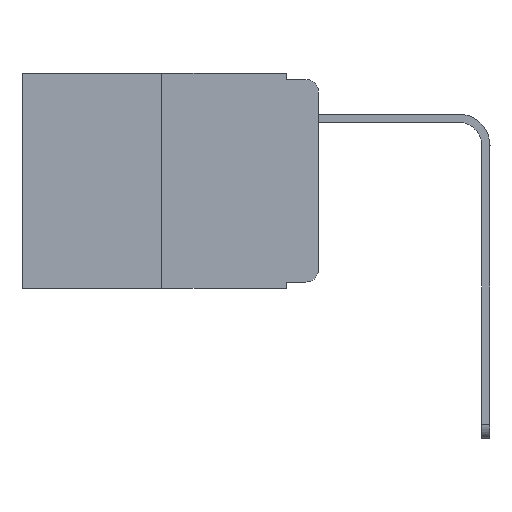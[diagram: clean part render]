
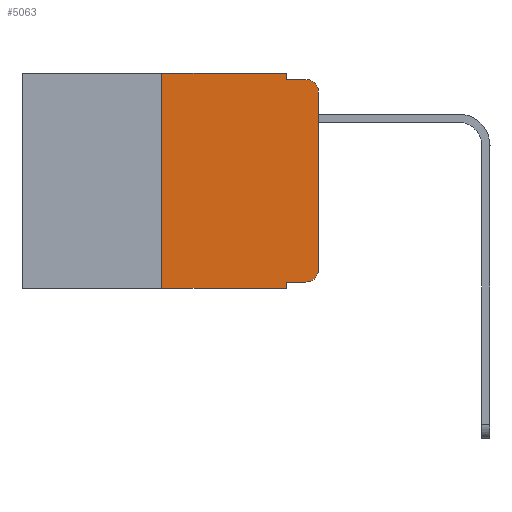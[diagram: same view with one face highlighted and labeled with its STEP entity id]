
A CAD part, left-side view. The second image highlights one B-rep face of the part: STEP entity #5063.
In plain terms, the highlighted planar face has unit normal (-1, 0, 0).
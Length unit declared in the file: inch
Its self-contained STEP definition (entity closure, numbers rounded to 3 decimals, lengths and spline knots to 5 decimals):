
#220 = CARTESIAN_POINT ( 'NONE',  ( 0., 0.25, 0. ) ) ;
#316 = DIRECTION ( 'NONE',  ( 0., 0., -1. ) ) ;
#384 = ORIENTED_EDGE ( 'NONE', *, *, #5271, .F. ) ;
#535 = VERTEX_POINT ( 'NONE', #10327 ) ;
#571 = EDGE_CURVE ( 'NONE', #6502, #5930, #3643, .T. ) ;
#575 = ORIENTED_EDGE ( 'NONE', *, *, #2331, .F. ) ;
#621 = DIRECTION ( 'NONE',  ( 0., 0., 1. ) ) ;
#719 = DIRECTION ( 'NONE',  ( -1., 0., 0. ) ) ;
#898 = CARTESIAN_POINT ( 'NONE',  ( 0., 0., -0.03 ) ) ;
#991 = EDGE_CURVE ( 'NONE', #1486, #1157, #9545, .T. ) ;
#1157 = VERTEX_POINT ( 'NONE', #9462 ) ;
#1486 = VERTEX_POINT ( 'NONE', #9009 ) ;
#1503 = CARTESIAN_POINT ( 'NONE',  ( 0., 0.473, 0. ) ) ;
#1522 = ORIENTED_EDGE ( 'NONE', *, *, #10848, .T. ) ;
#1525 = AXIS2_PLACEMENT_3D ( 'NONE', #6087, #719, #6989 ) ;
#1906 = VECTOR ( 'NONE', #10087, 39.37008 ) ;
#1943 = CIRCLE ( 'NONE', #1525, 0.02 ) ;
#1952 = ORIENTED_EDGE ( 'NONE', *, *, #8018, .F. ) ;
#2265 = EDGE_LOOP ( 'NONE', ( #9313, #9713, #575, #384, #1952, #3880, #11541, #6491, #1522, #4829 ) ) ;
#2331 = EDGE_CURVE ( 'NONE', #7788, #9104, #4872, .T. ) ;
#2636 = VECTOR ( 'NONE', #10453, 39.37008 ) ;
#2656 = VECTOR ( 'NONE', #4838, 39.37008 ) ;
#2702 = PLANE ( 'NONE',  #6130 ) ;
#3017 = VERTEX_POINT ( 'NONE', #6590 ) ;
#3643 = LINE ( 'NONE', #5897, #4207 ) ;
#3785 = CARTESIAN_POINT ( 'NONE',  ( 0., 0., 0. ) ) ;
#3832 = EDGE_CURVE ( 'NONE', #1157, #10319, #10558, .T. ) ;
#3880 = ORIENTED_EDGE ( 'NONE', *, *, #571, .F. ) ;
#3940 = CARTESIAN_POINT ( 'NONE',  ( 0., 0.051, -0.01 ) ) ;
#4207 = VECTOR ( 'NONE', #621, 39.37008 ) ;
#4244 = VECTOR ( 'NONE', #10772, 39.37008 ) ;
#4511 = CARTESIAN_POINT ( 'NONE',  ( 0., 0.02, -0.01 ) ) ;
#4617 = FACE_OUTER_BOUND ( 'NONE', #2265, .T. ) ;
#4671 = VECTOR ( 'NONE', #11520, 39.37008 ) ;
#4796 = CARTESIAN_POINT ( 'NONE',  ( 0., 0.02, -0.313 ) ) ;
#4829 = ORIENTED_EDGE ( 'NONE', *, *, #991, .T. ) ;
#4838 = DIRECTION ( 'NONE',  ( 0., 0., -1. ) ) ;
#4872 = LINE ( 'NONE', #3940, #9363 ) ;
#5039 = AXIS2_PLACEMENT_3D ( 'NONE', #4796, #9378, #316 ) ;
#5063 = ADVANCED_FACE ( 'NONE', ( #4617 ), #2702, .F. ) ;
#5271 = EDGE_CURVE ( 'NONE', #6372, #7788, #7131, .T. ) ;
#5481 = DIRECTION ( 'NONE',  ( 1., 0., 0. ) ) ;
#5635 = CARTESIAN_POINT ( 'NONE',  ( 0., 0.051, -0.01 ) ) ;
#5897 = CARTESIAN_POINT ( 'NONE',  ( 0., 0.25, 0. ) ) ;
#5930 = VERTEX_POINT ( 'NONE', #220 ) ;
#6087 = CARTESIAN_POINT ( 'NONE',  ( 0., 0.02, -0.03 ) ) ;
#6130 = AXIS2_PLACEMENT_3D ( 'NONE', #9925, #5481, #7226 ) ;
#6372 = VERTEX_POINT ( 'NONE', #9678 ) ;
#6491 = ORIENTED_EDGE ( 'NONE', *, *, #9301, .F. ) ;
#6502 = VERTEX_POINT ( 'NONE', #9881 ) ;
#6590 = CARTESIAN_POINT ( 'NONE',  ( 0., 0.051, -0.343 ) ) ;
#6605 = LINE ( 'NONE', #9003, #4244 ) ;
#6625 = DIRECTION ( 'NONE',  ( 0., -1., 0. ) ) ;
#6756 = LINE ( 'NONE', #7015, #4671 ) ;
#6772 = DIRECTION ( 'NONE',  ( 0., 0., 1. ) ) ;
#6989 = DIRECTION ( 'NONE',  ( 0., 0., -1. ) ) ;
#7015 = CARTESIAN_POINT ( 'NONE',  ( 0., 0.051, -0.333 ) ) ;
#7131 = LINE ( 'NONE', #8568, #2656 ) ;
#7226 = DIRECTION ( 'NONE',  ( 0., 0., -1. ) ) ;
#7788 = VERTEX_POINT ( 'NONE', #5635 ) ;
#8018 = EDGE_CURVE ( 'NONE', #5930, #6372, #8818, .T. ) ;
#8176 = EDGE_CURVE ( 'NONE', #10319, #9104, #1943, .T. ) ;
#8568 = CARTESIAN_POINT ( 'NONE',  ( 0., 0.051, 0. ) ) ;
#8818 = LINE ( 'NONE', #1503, #2636 ) ;
#9003 = CARTESIAN_POINT ( 'NONE',  ( 0., 0.473, -0.343 ) ) ;
#9009 = CARTESIAN_POINT ( 'NONE',  ( 0., 0.02, -0.333 ) ) ;
#9104 = VERTEX_POINT ( 'NONE', #4511 ) ;
#9253 = CARTESIAN_POINT ( 'NONE',  ( 0., 0.051, 0. ) ) ;
#9301 = EDGE_CURVE ( 'NONE', #535, #3017, #10320, .T. ) ;
#9313 = ORIENTED_EDGE ( 'NONE', *, *, #3832, .T. ) ;
#9363 = VECTOR ( 'NONE', #6625, 39.37008 ) ;
#9378 = DIRECTION ( 'NONE',  ( -1., 0., 0. ) ) ;
#9462 = CARTESIAN_POINT ( 'NONE',  ( 0., 0., -0.313 ) ) ;
#9545 = CIRCLE ( 'NONE', #5039, 0.02 ) ;
#9580 = VECTOR ( 'NONE', #6772, 39.37008 ) ;
#9678 = CARTESIAN_POINT ( 'NONE',  ( 0., 0.051, 0. ) ) ;
#9713 = ORIENTED_EDGE ( 'NONE', *, *, #8176, .T. ) ;
#9881 = CARTESIAN_POINT ( 'NONE',  ( 0., 0.25, -0.343 ) ) ;
#9925 = CARTESIAN_POINT ( 'NONE',  ( 0., 0.473, 0. ) ) ;
#10087 = DIRECTION ( 'NONE',  ( 0., 0., -1. ) ) ;
#10319 = VERTEX_POINT ( 'NONE', #898 ) ;
#10320 = LINE ( 'NONE', #9253, #1906 ) ;
#10327 = CARTESIAN_POINT ( 'NONE',  ( 0., 0.051, -0.333 ) ) ;
#10453 = DIRECTION ( 'NONE',  ( 0., -1., 0. ) ) ;
#10558 = LINE ( 'NONE', #3785, #9580 ) ;
#10772 = DIRECTION ( 'NONE',  ( 0., -1., 0. ) ) ;
#10848 = EDGE_CURVE ( 'NONE', #535, #1486, #6756, .T. ) ;
#11520 = DIRECTION ( 'NONE',  ( 0., -1., 0. ) ) ;
#11541 = ORIENTED_EDGE ( 'NONE', *, *, #11551, .T. ) ;
#11551 = EDGE_CURVE ( 'NONE', #6502, #3017, #6605, .T. ) ;
